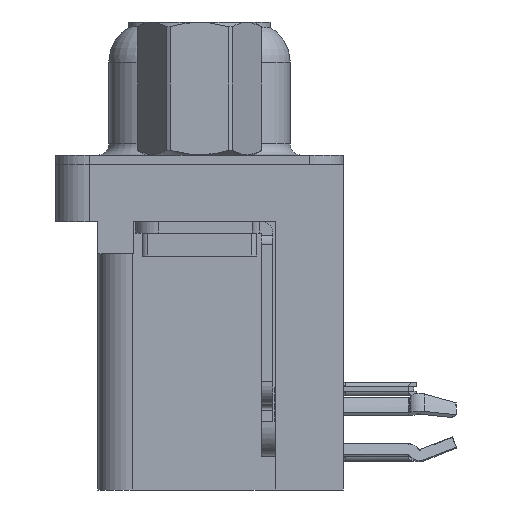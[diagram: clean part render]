
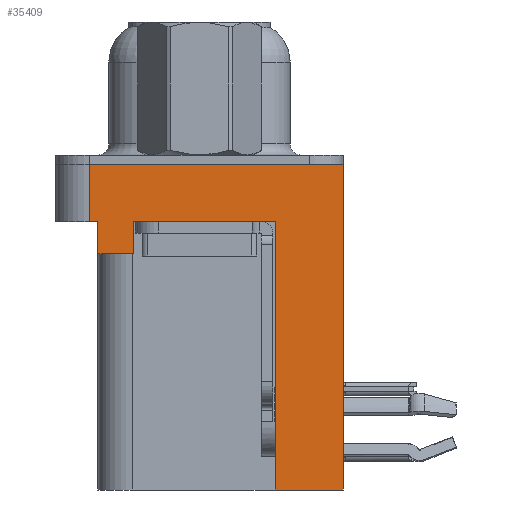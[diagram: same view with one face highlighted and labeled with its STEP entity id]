
A CAD part, left-side view. The second image highlights one B-rep face of the part: STEP entity #35409.
In plain terms, the highlighted planar face has unit normal (-1, 0, 0).
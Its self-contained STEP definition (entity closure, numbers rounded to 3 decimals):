
#82 = DIRECTION ( 'NONE',  ( 0., -1., 0. ) ) ;
#756 = EDGE_CURVE ( 'NONE', #16241, #2918, #12168, .T. ) ;
#795 = CARTESIAN_POINT ( 'NONE',  ( -2.91, 4.425, -3.9 ) ) ;
#801 = CARTESIAN_POINT ( 'NONE',  ( -2.91, -3.295, -14.2 ) ) ;
#1006 = LINE ( 'NONE', #4065, #33071 ) ;
#1408 = ORIENTED_EDGE ( 'NONE', *, *, #28030, .F. ) ;
#2006 = DIRECTION ( 'NONE',  ( -1., 0., 0. ) ) ;
#2182 = CARTESIAN_POINT ( 'NONE',  ( -2.91, -3.295, -14.2 ) ) ;
#2918 = VERTEX_POINT ( 'NONE', #40291 ) ;
#3195 = EDGE_CURVE ( 'NONE', #37287, #42027, #19639, .T. ) ;
#3561 = LINE ( 'NONE', #36349, #16042 ) ;
#4065 = CARTESIAN_POINT ( 'NONE',  ( -2.91, 4.775, -2.5 ) ) ;
#4721 = LINE ( 'NONE', #801, #12707 ) ;
#5659 = DIRECTION ( 'NONE',  ( 0., 0., 1. ) ) ;
#6626 = VECTOR ( 'NONE', #5659, 1000. ) ;
#7435 = LINE ( 'NONE', #25423, #9422 ) ;
#7742 = DIRECTION ( 'NONE',  ( 0., 0., 1. ) ) ;
#7784 = ORIENTED_EDGE ( 'NONE', *, *, #3195, .F. ) ;
#7939 = VECTOR ( 'NONE', #11981, 1000. ) ;
#7951 = LINE ( 'NONE', #795, #19895 ) ;
#9422 = VECTOR ( 'NONE', #38664, 1000. ) ;
#10047 = DIRECTION ( 'NONE',  ( 0., -1., 0. ) ) ;
#10576 = DIRECTION ( 'NONE',  ( 0., 1., 0. ) ) ;
#11468 = VERTEX_POINT ( 'NONE', #14292 ) ;
#11981 = DIRECTION ( 'NONE',  ( 0., 1., 0. ) ) ;
#11990 = PLANE ( 'NONE',  #42086 ) ;
#12168 = LINE ( 'NONE', #2182, #6626 ) ;
#12209 = FACE_OUTER_BOUND ( 'NONE', #34980, .T. ) ;
#12438 = CARTESIAN_POINT ( 'NONE',  ( -2.91, -6.275, -2.5 ) ) ;
#12707 = VECTOR ( 'NONE', #10576, 1000. ) ;
#12768 = CARTESIAN_POINT ( 'NONE',  ( -2.91, 2.895, -2.5 ) ) ;
#13887 = LINE ( 'NONE', #40821, #25254 ) ;
#14141 = EDGE_CURVE ( 'NONE', #24980, #42027, #7435, .T. ) ;
#14155 = ORIENTED_EDGE ( 'NONE', *, *, #25742, .T. ) ;
#14292 = CARTESIAN_POINT ( 'NONE',  ( -2.91, 4.425, -2.5 ) ) ;
#14786 = ORIENTED_EDGE ( 'NONE', *, *, #14141, .T. ) ;
#15442 = DIRECTION ( 'NONE',  ( 0., -1., 0. ) ) ;
#16042 = VECTOR ( 'NONE', #82, 1000. ) ;
#16168 = CARTESIAN_POINT ( 'NONE',  ( -2.91, 4.775, 0. ) ) ;
#16241 = VERTEX_POINT ( 'NONE', #19723 ) ;
#16729 = VERTEX_POINT ( 'NONE', #31309 ) ;
#17932 = VECTOR ( 'NONE', #15442, 1000. ) ;
#18709 = CARTESIAN_POINT ( 'NONE',  ( -2.91, 4.425, -3.9 ) ) ;
#19490 = ORIENTED_EDGE ( 'NONE', *, *, #30324, .F. ) ;
#19639 = LINE ( 'NONE', #32889, #40770 ) ;
#19723 = CARTESIAN_POINT ( 'NONE',  ( -2.91, -3.295, -14.2 ) ) ;
#19895 = VECTOR ( 'NONE', #7742, 1000. ) ;
#20175 = CARTESIAN_POINT ( 'NONE',  ( -2.91, 4.425, -3.9 ) ) ;
#20250 = EDGE_CURVE ( 'NONE', #38439, #2918, #28923, .T. ) ;
#20790 = DIRECTION ( 'NONE',  ( 0., 0., 1. ) ) ;
#23132 = ORIENTED_EDGE ( 'NONE', *, *, #756, .F. ) ;
#23480 = ORIENTED_EDGE ( 'NONE', *, *, #29513, .T. ) ;
#24119 = ORIENTED_EDGE ( 'NONE', *, *, #20250, .T. ) ;
#24324 = DIRECTION ( 'NONE',  ( 0., 0., 1. ) ) ;
#24708 = CARTESIAN_POINT ( 'NONE',  ( -2.91, -6.275, -14.2 ) ) ;
#24980 = VERTEX_POINT ( 'NONE', #24708 ) ;
#25254 = VECTOR ( 'NONE', #24324, 1000. ) ;
#25423 = CARTESIAN_POINT ( 'NONE',  ( -2.91, -6.275, -2.5 ) ) ;
#25469 = DIRECTION ( 'NONE',  ( 0., 0., 1. ) ) ;
#25742 = EDGE_CURVE ( 'NONE', #16729, #11468, #3561, .T. ) ;
#28030 = EDGE_CURVE ( 'NONE', #24980, #16241, #4721, .T. ) ;
#28923 = LINE ( 'NONE', #35855, #17932 ) ;
#29513 = EDGE_CURVE ( 'NONE', #31925, #38439, #13887, .T. ) ;
#30324 = EDGE_CURVE ( 'NONE', #31925, #39673, #41744, .T. ) ;
#30790 = CARTESIAN_POINT ( 'NONE',  ( -2.91, 2.895, -3.9 ) ) ;
#31309 = CARTESIAN_POINT ( 'NONE',  ( -2.91, 4.775, -2.5 ) ) ;
#31925 = VERTEX_POINT ( 'NONE', #30790 ) ;
#32889 = CARTESIAN_POINT ( 'NONE',  ( -2.91, -6.275, 0. ) ) ;
#32908 = CARTESIAN_POINT ( 'NONE',  ( -2.91, -6.275, 0. ) ) ;
#33071 = VECTOR ( 'NONE', #20790, 1000. ) ;
#33825 = ORIENTED_EDGE ( 'NONE', *, *, #35197, .F. ) ;
#34980 = EDGE_LOOP ( 'NONE', ( #7784, #40887, #14155, #33825, #19490, #23480, #24119, #23132, #1408, #14786 ) ) ;
#35186 = EDGE_CURVE ( 'NONE', #16729, #37287, #1006, .T. ) ;
#35197 = EDGE_CURVE ( 'NONE', #39673, #11468, #7951, .T. ) ;
#35409 = ADVANCED_FACE ( 'NONE', ( #12209 ), #11990, .T. ) ;
#35855 = CARTESIAN_POINT ( 'NONE',  ( -2.91, -6.275, -2.5 ) ) ;
#36349 = CARTESIAN_POINT ( 'NONE',  ( -2.91, -6.275, -2.5 ) ) ;
#37287 = VERTEX_POINT ( 'NONE', #16168 ) ;
#38439 = VERTEX_POINT ( 'NONE', #12768 ) ;
#38664 = DIRECTION ( 'NONE',  ( 0., 0., 1. ) ) ;
#39673 = VERTEX_POINT ( 'NONE', #20175 ) ;
#40291 = CARTESIAN_POINT ( 'NONE',  ( -2.91, -3.295, -2.5 ) ) ;
#40770 = VECTOR ( 'NONE', #10047, 1000. ) ;
#40821 = CARTESIAN_POINT ( 'NONE',  ( -2.91, 2.895, -3.9 ) ) ;
#40887 = ORIENTED_EDGE ( 'NONE', *, *, #35186, .F. ) ;
#41744 = LINE ( 'NONE', #18709, #7939 ) ;
#42027 = VERTEX_POINT ( 'NONE', #32908 ) ;
#42086 = AXIS2_PLACEMENT_3D ( 'NONE', #12438, #2006, #25469 ) ;
